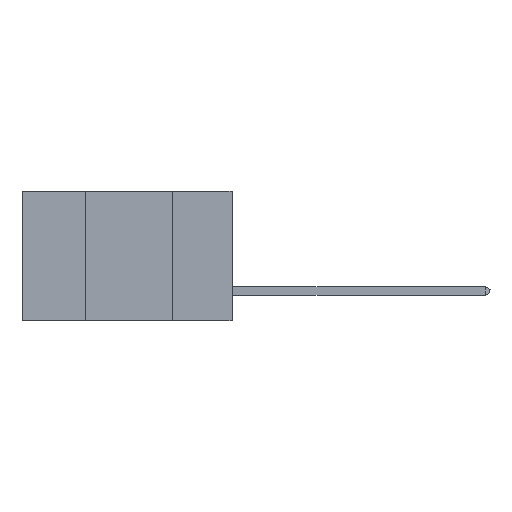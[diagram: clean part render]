
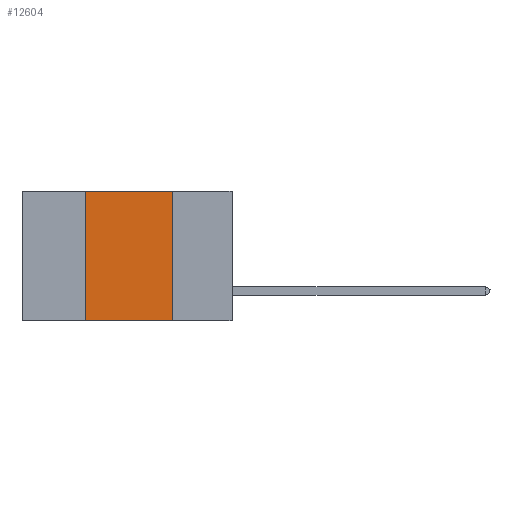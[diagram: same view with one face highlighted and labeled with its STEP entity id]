
A CAD part, left-side view. The second image highlights one B-rep face of the part: STEP entity #12604.
In plain terms, the highlighted planar face has unit normal (-1, 0, 0).
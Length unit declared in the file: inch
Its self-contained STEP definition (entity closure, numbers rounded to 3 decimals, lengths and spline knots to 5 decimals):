
#45 = EDGE_LOOP ( 'NONE', ( #6965, #11931, #1118, #2616 ) ) ;
#79 = LINE ( 'NONE', #13394, #9394 ) ;
#231 = CARTESIAN_POINT ( 'NONE',  ( 0., 0.17, 0. ) ) ;
#1118 = ORIENTED_EDGE ( 'NONE', *, *, #6255, .F. ) ;
#1419 = EDGE_CURVE ( 'NONE', #6162, #9903, #9960, .T. ) ;
#2110 = DIRECTION ( 'NONE',  ( 0., -1., 0. ) ) ;
#2147 = CARTESIAN_POINT ( 'NONE',  ( 0., 0.42, -0.37 ) ) ;
#2616 = ORIENTED_EDGE ( 'NONE', *, *, #12718, .T. ) ;
#3448 = VECTOR ( 'NONE', #10724, 39.37008 ) ;
#3868 = DIRECTION ( 'NONE',  ( 1., 0., 0. ) ) ;
#5061 = CARTESIAN_POINT ( 'NONE',  ( 0., 0.6, 0. ) ) ;
#5437 = VERTEX_POINT ( 'NONE', #2147 ) ;
#6162 = VERTEX_POINT ( 'NONE', #14393 ) ;
#6255 = EDGE_CURVE ( 'NONE', #5437, #6162, #79, .T. ) ;
#6303 = DIRECTION ( 'NONE',  ( 0., 0., -1. ) ) ;
#6316 = FACE_OUTER_BOUND ( 'NONE', #45, .T. ) ;
#6965 = ORIENTED_EDGE ( 'NONE', *, *, #7994, .F. ) ;
#7239 = LINE ( 'NONE', #11614, #7838 ) ;
#7312 = DIRECTION ( 'NONE',  ( 0., 0., 1. ) ) ;
#7581 = DIRECTION ( 'NONE',  ( 0., 0., -1. ) ) ;
#7838 = VECTOR ( 'NONE', #2110, 39.37008 ) ;
#7994 = EDGE_CURVE ( 'NONE', #9903, #10969, #15465, .T. ) ;
#7997 = CARTESIAN_POINT ( 'NONE',  ( 0., 0.17, 0. ) ) ;
#9394 = VECTOR ( 'NONE', #7312, 39.37008 ) ;
#9903 = VERTEX_POINT ( 'NONE', #7997 ) ;
#9960 = LINE ( 'NONE', #15516, #3448 ) ;
#9965 = PLANE ( 'NONE',  #11343 ) ;
#10724 = DIRECTION ( 'NONE',  ( 0., -1., 0. ) ) ;
#10969 = VERTEX_POINT ( 'NONE', #13411 ) ;
#11343 = AXIS2_PLACEMENT_3D ( 'NONE', #5061, #3868, #7581 ) ;
#11562 = VECTOR ( 'NONE', #6303, 39.37008 ) ;
#11614 = CARTESIAN_POINT ( 'NONE',  ( 0., 0.6, -0.37 ) ) ;
#11931 = ORIENTED_EDGE ( 'NONE', *, *, #1419, .F. ) ;
#12604 = ADVANCED_FACE ( 'NONE', ( #6316 ), #9965, .F. ) ;
#12718 = EDGE_CURVE ( 'NONE', #5437, #10969, #7239, .T. ) ;
#13394 = CARTESIAN_POINT ( 'NONE',  ( 0., 0.42, 0. ) ) ;
#13411 = CARTESIAN_POINT ( 'NONE',  ( 0., 0.17, -0.37 ) ) ;
#14393 = CARTESIAN_POINT ( 'NONE',  ( 0., 0.42, 0. ) ) ;
#15465 = LINE ( 'NONE', #231, #11562 ) ;
#15516 = CARTESIAN_POINT ( 'NONE',  ( 0., 0.6, 0. ) ) ;
